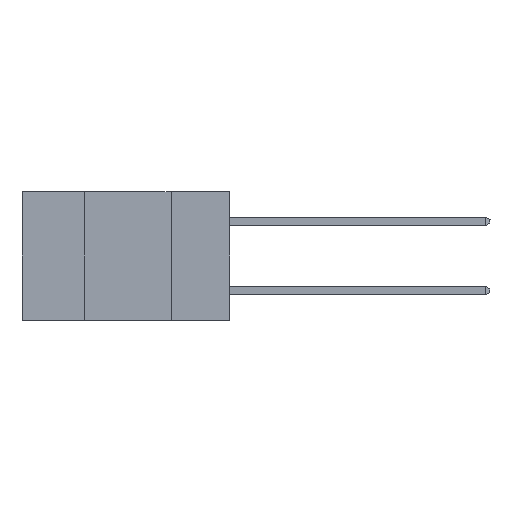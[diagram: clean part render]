
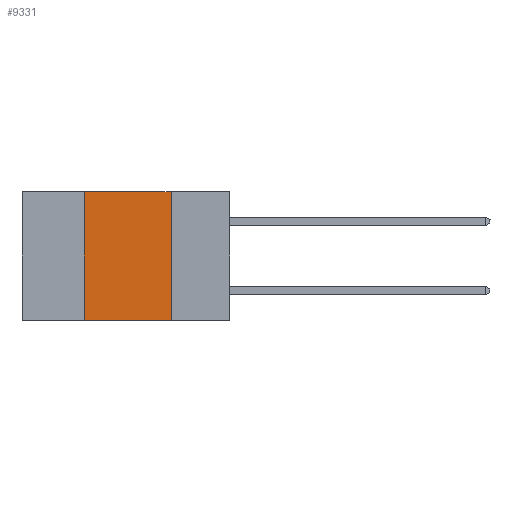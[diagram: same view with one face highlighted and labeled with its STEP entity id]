
A CAD part, left-side view. The second image highlights one B-rep face of the part: STEP entity #9331.
In plain terms, the highlighted planar face has unit normal (-1, 0, 0).
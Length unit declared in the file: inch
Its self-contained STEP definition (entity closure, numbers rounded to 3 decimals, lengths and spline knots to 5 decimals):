
#122 = CARTESIAN_POINT ( 'NONE',  ( 0., 0.42, -0.37 ) ) ;
#947 = PLANE ( 'NONE',  #3800 ) ;
#1335 = CARTESIAN_POINT ( 'NONE',  ( 0., 0.6, 0. ) ) ;
#1912 = CARTESIAN_POINT ( 'NONE',  ( 0., 0.17, -0.37 ) ) ;
#2095 = FACE_OUTER_BOUND ( 'NONE', #6985, .T. ) ;
#2100 = ORIENTED_EDGE ( 'NONE', *, *, #2627, .F. ) ;
#2165 = DIRECTION ( 'NONE',  ( 1., 0., 0. ) ) ;
#2270 = CARTESIAN_POINT ( 'NONE',  ( 0., 0.17, 0. ) ) ;
#2290 = EDGE_CURVE ( 'NONE', #2464, #7900, #9483, .T. ) ;
#2464 = VERTEX_POINT ( 'NONE', #12929 ) ;
#2568 = EDGE_CURVE ( 'NONE', #2464, #6101, #10289, .T. ) ;
#2627 = EDGE_CURVE ( 'NONE', #6469, #6101, #12262, .T. ) ;
#3800 = AXIS2_PLACEMENT_3D ( 'NONE', #10337, #2165, #9126 ) ;
#4443 = LINE ( 'NONE', #1335, #12249 ) ;
#4587 = ORIENTED_EDGE ( 'NONE', *, *, #11261, .F. ) ;
#4700 = VECTOR ( 'NONE', #12531, 39.37008 ) ;
#6101 = VERTEX_POINT ( 'NONE', #1912 ) ;
#6469 = VERTEX_POINT ( 'NONE', #2270 ) ;
#6985 = EDGE_LOOP ( 'NONE', ( #2100, #4587, #13300, #8543 ) ) ;
#7002 = CARTESIAN_POINT ( 'NONE',  ( 0., 0.17, -0.37 ) ) ;
#7900 = VERTEX_POINT ( 'NONE', #12304 ) ;
#8283 = VECTOR ( 'NONE', #9143, 39.37008 ) ;
#8543 = ORIENTED_EDGE ( 'NONE', *, *, #2568, .T. ) ;
#9085 = DIRECTION ( 'NONE',  ( 0., -1., 0. ) ) ;
#9126 = DIRECTION ( 'NONE',  ( 0., 0., -1. ) ) ;
#9143 = DIRECTION ( 'NONE',  ( 0., 0., -1. ) ) ;
#9331 = ADVANCED_FACE ( 'NONE', ( #2095 ), #947, .F. ) ;
#9483 = LINE ( 'NONE', #122, #4700 ) ;
#10160 = CARTESIAN_POINT ( 'NONE',  ( 0., 0.6, -0.37 ) ) ;
#10289 = LINE ( 'NONE', #10160, #12593 ) ;
#10337 = CARTESIAN_POINT ( 'NONE',  ( 0., 0.6, 0. ) ) ;
#10525 = DIRECTION ( 'NONE',  ( 0., -1., 0. ) ) ;
#11261 = EDGE_CURVE ( 'NONE', #7900, #6469, #4443, .T. ) ;
#12249 = VECTOR ( 'NONE', #10525, 39.37008 ) ;
#12262 = LINE ( 'NONE', #7002, #8283 ) ;
#12304 = CARTESIAN_POINT ( 'NONE',  ( 0., 0.42, 0. ) ) ;
#12531 = DIRECTION ( 'NONE',  ( 0., 0., 1. ) ) ;
#12593 = VECTOR ( 'NONE', #9085, 39.37008 ) ;
#12929 = CARTESIAN_POINT ( 'NONE',  ( 0., 0.42, -0.37 ) ) ;
#13300 = ORIENTED_EDGE ( 'NONE', *, *, #2290, .F. ) ;
